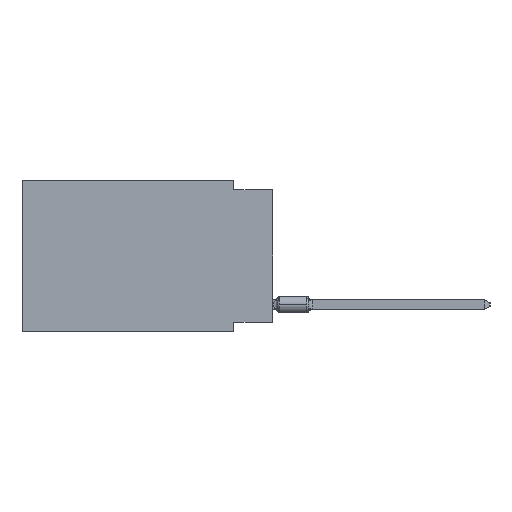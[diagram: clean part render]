
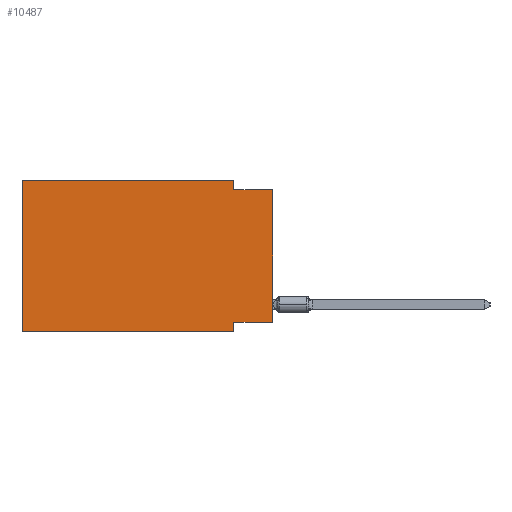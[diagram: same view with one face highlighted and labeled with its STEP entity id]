
A CAD part, left-side view. The second image highlights one B-rep face of the part: STEP entity #10487.
In plain terms, the highlighted planar face has unit normal (-1, 0, 0).
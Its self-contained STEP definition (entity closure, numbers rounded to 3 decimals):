
#996 = VECTOR ( 'NONE', #25693, 1000. ) ;
#1003 = DIRECTION ( 'NONE',  ( 0., 0., 1. ) ) ;
#1472 = ORIENTED_EDGE ( 'NONE', *, *, #2804, .T. ) ;
#2171 = VECTOR ( 'NONE', #32207, 1000. ) ;
#2179 = VERTEX_POINT ( 'NONE', #19978 ) ;
#2804 = EDGE_CURVE ( 'NONE', #2179, #27329, #27842, .T. ) ;
#3321 = CARTESIAN_POINT ( 'NONE',  ( 0., 2.54, -9.271 ) ) ;
#3632 = DIRECTION ( 'NONE',  ( 1., 0., 0. ) ) ;
#4598 = ORIENTED_EDGE ( 'NONE', *, *, #26464, .T. ) ;
#6337 = EDGE_CURVE ( 'NONE', #43985, #33763, #7412, .T. ) ;
#7412 = LINE ( 'NONE', #21514, #35419 ) ;
#8692 = CARTESIAN_POINT ( 'NONE',  ( 0., 2.54, -9.906 ) ) ;
#9026 = EDGE_CURVE ( 'NONE', #44392, #25873, #34925, .T. ) ;
#9466 = DIRECTION ( 'NONE',  ( 0., -1., 0. ) ) ;
#10487 = ADVANCED_FACE ( 'NONE', ( #41927 ), #38723, .F. ) ;
#11389 = ORIENTED_EDGE ( 'NONE', *, *, #9026, .F. ) ;
#11597 = CARTESIAN_POINT ( 'NONE',  ( 0., 0., 0. ) ) ;
#12087 = CARTESIAN_POINT ( 'NONE',  ( 0., 16.383, 0. ) ) ;
#12108 = ORIENTED_EDGE ( 'NONE', *, *, #23160, .F. ) ;
#13537 = CARTESIAN_POINT ( 'NONE',  ( 0., 2.54, 0. ) ) ;
#14641 = EDGE_CURVE ( 'NONE', #26519, #31749, #37153, .T. ) ;
#15457 = VECTOR ( 'NONE', #9466, 1000. ) ;
#16357 = ORIENTED_EDGE ( 'NONE', *, *, #32500, .F. ) ;
#17491 = DIRECTION ( 'NONE',  ( 0., 0., -1. ) ) ;
#18132 = LINE ( 'NONE', #45325, #2171 ) ;
#19135 = VECTOR ( 'NONE', #1003, 1000. ) ;
#19249 = LINE ( 'NONE', #12087, #19135 ) ;
#19401 = CARTESIAN_POINT ( 'NONE',  ( 0., 16.383, 0. ) ) ;
#19978 = CARTESIAN_POINT ( 'NONE',  ( 0., 16.383, -9.906 ) ) ;
#21129 = ORIENTED_EDGE ( 'NONE', *, *, #6337, .F. ) ;
#21514 = CARTESIAN_POINT ( 'NONE',  ( 0., 0., -0.635 ) ) ;
#23061 = ORIENTED_EDGE ( 'NONE', *, *, #32435, .F. ) ;
#23160 = EDGE_CURVE ( 'NONE', #25873, #27329, #27555, .T. ) ;
#25693 = DIRECTION ( 'NONE',  ( 0., 0., 1. ) ) ;
#25852 = CARTESIAN_POINT ( 'NONE',  ( 0., 0., -0.635 ) ) ;
#25873 = VERTEX_POINT ( 'NONE', #3321 ) ;
#26464 = EDGE_CURVE ( 'NONE', #44392, #33763, #36504, .T. ) ;
#26519 = VERTEX_POINT ( 'NONE', #43870 ) ;
#26687 = EDGE_LOOP ( 'NONE', ( #4598, #21129, #23061, #39259, #16357, #1472, #12108, #11389 ) ) ;
#27329 = VERTEX_POINT ( 'NONE', #8692 ) ;
#27555 = LINE ( 'NONE', #31700, #37602 ) ;
#27842 = LINE ( 'NONE', #42599, #28449 ) ;
#28351 = CARTESIAN_POINT ( 'NONE',  ( 0., 16.383, 0. ) ) ;
#28449 = VECTOR ( 'NONE', #41891, 1000. ) ;
#28663 = DIRECTION ( 'NONE',  ( 0., -1., 0. ) ) ;
#31044 = VECTOR ( 'NONE', #37476, 1000. ) ;
#31700 = CARTESIAN_POINT ( 'NONE',  ( 0., 2.54, -9.906 ) ) ;
#31749 = VERTEX_POINT ( 'NONE', #13537 ) ;
#32207 = DIRECTION ( 'NONE',  ( 0., 0., -1. ) ) ;
#32435 = EDGE_CURVE ( 'NONE', #31749, #43985, #18132, .T. ) ;
#32500 = EDGE_CURVE ( 'NONE', #2179, #26519, #19249, .T. ) ;
#32849 = AXIS2_PLACEMENT_3D ( 'NONE', #28351, #3632, #17491 ) ;
#33763 = VERTEX_POINT ( 'NONE', #25852 ) ;
#34045 = CARTESIAN_POINT ( 'NONE',  ( 0., 0., -9.271 ) ) ;
#34925 = LINE ( 'NONE', #34045, #31044 ) ;
#35419 = VECTOR ( 'NONE', #28663, 1000. ) ;
#35936 = CARTESIAN_POINT ( 'NONE',  ( 0., 0., -9.271 ) ) ;
#36504 = LINE ( 'NONE', #11597, #996 ) ;
#37153 = LINE ( 'NONE', #19401, #15457 ) ;
#37476 = DIRECTION ( 'NONE',  ( 0., 1., 0. ) ) ;
#37602 = VECTOR ( 'NONE', #42056, 1000. ) ;
#38723 = PLANE ( 'NONE',  #32849 ) ;
#39259 = ORIENTED_EDGE ( 'NONE', *, *, #14641, .F. ) ;
#41891 = DIRECTION ( 'NONE',  ( 0., -1., 0. ) ) ;
#41927 = FACE_OUTER_BOUND ( 'NONE', #26687, .T. ) ;
#42056 = DIRECTION ( 'NONE',  ( 0., 0., -1. ) ) ;
#42599 = CARTESIAN_POINT ( 'NONE',  ( 0., 16.383, -9.906 ) ) ;
#42727 = CARTESIAN_POINT ( 'NONE',  ( 0., 2.54, -0.635 ) ) ;
#43870 = CARTESIAN_POINT ( 'NONE',  ( 0., 16.383, 0. ) ) ;
#43985 = VERTEX_POINT ( 'NONE', #42727 ) ;
#44392 = VERTEX_POINT ( 'NONE', #35936 ) ;
#45325 = CARTESIAN_POINT ( 'NONE',  ( 0., 2.54, 0. ) ) ;
